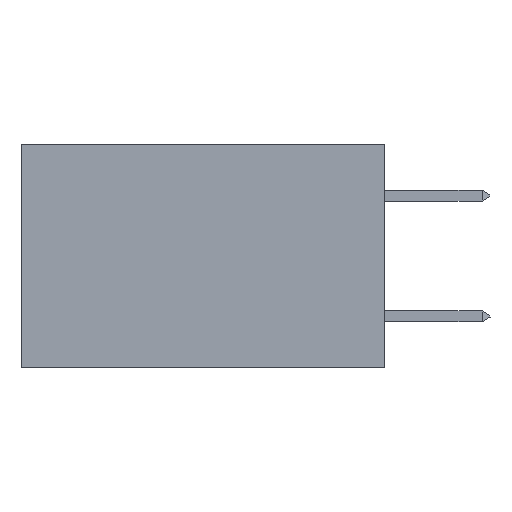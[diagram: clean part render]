
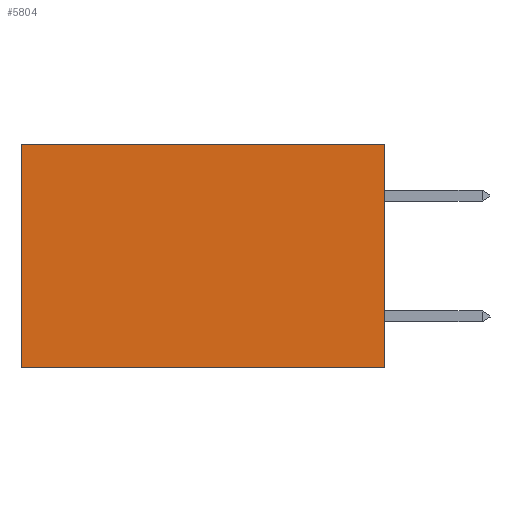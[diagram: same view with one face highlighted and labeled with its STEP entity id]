
A CAD part, left-side view. The second image highlights one B-rep face of the part: STEP entity #5804.
In plain terms, the highlighted planar face has unit normal (-1, 0, 0).
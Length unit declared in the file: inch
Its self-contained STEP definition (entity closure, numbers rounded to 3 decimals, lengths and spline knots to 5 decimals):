
#1389 = CARTESIAN_POINT ( 'NONE',  ( 0.2875, 0., 0. ) ) ;
#3284 = DIRECTION ( 'NONE',  ( 1., 0., 0. ) ) ;
#5804 = ADVANCED_FACE ( 'NONE', ( #28784 ), #6244, .F. ) ;
#6244 = PLANE ( 'NONE',  #34457 ) ;
#7089 = CARTESIAN_POINT ( 'NONE',  ( 0.2875, 0., 0. ) ) ;
#7650 = LINE ( 'NONE', #35607, #40501 ) ;
#8283 = LINE ( 'NONE', #12372, #24271 ) ;
#10616 = CARTESIAN_POINT ( 'NONE',  ( 0.2875, 0., -0.37 ) ) ;
#11748 = ORIENTED_EDGE ( 'NONE', *, *, #40590, .T. ) ;
#12372 = CARTESIAN_POINT ( 'NONE',  ( 0.2875, 0., -0.37 ) ) ;
#12602 = DIRECTION ( 'NONE',  ( 0., 0., -1. ) ) ;
#12636 = DIRECTION ( 'NONE',  ( 0., 1., 0. ) ) ;
#13709 = EDGE_CURVE ( 'NONE', #20956, #29364, #19580, .T. ) ;
#14121 = VERTEX_POINT ( 'NONE', #40357 ) ;
#15506 = EDGE_CURVE ( 'NONE', #20956, #31286, #33360, .T. ) ;
#18418 = ORIENTED_EDGE ( 'NONE', *, *, #15506, .T. ) ;
#19580 = LINE ( 'NONE', #38320, #30042 ) ;
#20956 = VERTEX_POINT ( 'NONE', #7089 ) ;
#22701 = DIRECTION ( 'NONE',  ( 0., 0., -1. ) ) ;
#24271 = VECTOR ( 'NONE', #12636, 39.37008 ) ;
#26510 = ORIENTED_EDGE ( 'NONE', *, *, #30375, .F. ) ;
#26922 = ORIENTED_EDGE ( 'NONE', *, *, #13709, .F. ) ;
#28784 = FACE_OUTER_BOUND ( 'NONE', #41202, .T. ) ;
#29364 = VERTEX_POINT ( 'NONE', #10616 ) ;
#30042 = VECTOR ( 'NONE', #12602, 39.37008 ) ;
#30375 = EDGE_CURVE ( 'NONE', #29364, #14121, #8283, .T. ) ;
#31286 = VERTEX_POINT ( 'NONE', #34198 ) ;
#32379 = VECTOR ( 'NONE', #39835, 39.37008 ) ;
#33360 = LINE ( 'NONE', #1389, #32379 ) ;
#34198 = CARTESIAN_POINT ( 'NONE',  ( 0.2875, 0.6, 0. ) ) ;
#34457 = AXIS2_PLACEMENT_3D ( 'NONE', #34814, #3284, #35367 ) ;
#34814 = CARTESIAN_POINT ( 'NONE',  ( 0.2875, 0., 0. ) ) ;
#35367 = DIRECTION ( 'NONE',  ( 0., 0., -1. ) ) ;
#35607 = CARTESIAN_POINT ( 'NONE',  ( 0.2875, 0.6, 0. ) ) ;
#38320 = CARTESIAN_POINT ( 'NONE',  ( 0.2875, 0., 0. ) ) ;
#39835 = DIRECTION ( 'NONE',  ( 0., 1., 0. ) ) ;
#40357 = CARTESIAN_POINT ( 'NONE',  ( 0.2875, 0.6, -0.37 ) ) ;
#40501 = VECTOR ( 'NONE', #22701, 39.37008 ) ;
#40590 = EDGE_CURVE ( 'NONE', #31286, #14121, #7650, .T. ) ;
#41202 = EDGE_LOOP ( 'NONE', ( #11748, #26510, #26922, #18418 ) ) ;
